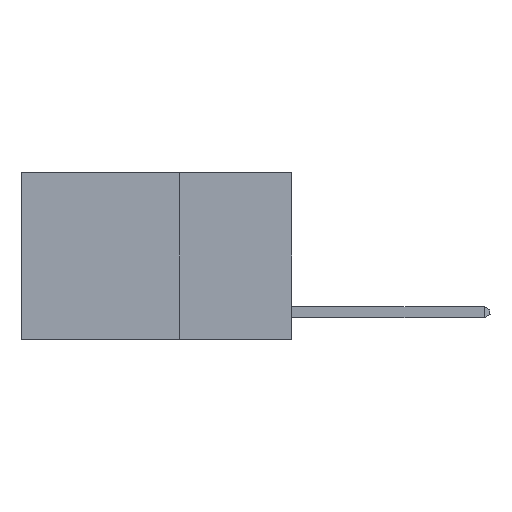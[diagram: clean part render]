
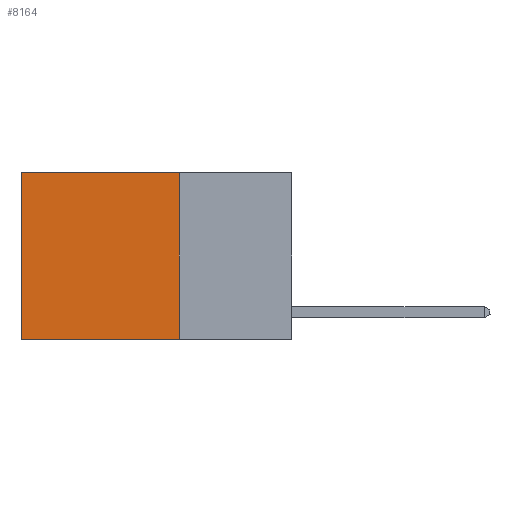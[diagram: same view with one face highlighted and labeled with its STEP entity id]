
A CAD part, left-side view. The second image highlights one B-rep face of the part: STEP entity #8164.
In plain terms, the highlighted planar face has unit normal (-1, 0, 0).
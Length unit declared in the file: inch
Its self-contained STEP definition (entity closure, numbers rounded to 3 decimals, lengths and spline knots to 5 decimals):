
#120 = VERTEX_POINT ( 'NONE', #10152 ) ;
#177 = VECTOR ( 'NONE', #1969, 39.37008 ) ;
#361 = VECTOR ( 'NONE', #2943, 39.37008 ) ;
#1296 = AXIS2_PLACEMENT_3D ( 'NONE', #7259, #12402, #7137 ) ;
#1969 = DIRECTION ( 'NONE',  ( 0., 0., -1. ) ) ;
#2112 = EDGE_CURVE ( 'NONE', #12924, #120, #5916, .T. ) ;
#2836 = DIRECTION ( 'NONE',  ( 0., 1., 0. ) ) ;
#2943 = DIRECTION ( 'NONE',  ( 0., 0., -1. ) ) ;
#3273 = EDGE_LOOP ( 'NONE', ( #9702, #4408, #4881, #5681 ) ) ;
#4176 = EDGE_CURVE ( 'NONE', #7712, #12924, #6089, .T. ) ;
#4379 = CARTESIAN_POINT ( 'NONE',  ( 0.2625, 0.25, 0. ) ) ;
#4408 = ORIENTED_EDGE ( 'NONE', *, *, #2112, .F. ) ;
#4881 = ORIENTED_EDGE ( 'NONE', *, *, #4176, .F. ) ;
#5681 = ORIENTED_EDGE ( 'NONE', *, *, #9122, .T. ) ;
#5916 = LINE ( 'NONE', #12054, #6511 ) ;
#6089 = LINE ( 'NONE', #12163, #361 ) ;
#6100 = CARTESIAN_POINT ( 'NONE',  ( 0.2625, 0.6, 0. ) ) ;
#6511 = VECTOR ( 'NONE', #2836, 39.37008 ) ;
#7137 = DIRECTION ( 'NONE',  ( 0., 0., -1. ) ) ;
#7259 = CARTESIAN_POINT ( 'NONE',  ( 0.2625, 0.25, 0. ) ) ;
#7391 = EDGE_CURVE ( 'NONE', #9214, #120, #10397, .T. ) ;
#7712 = VERTEX_POINT ( 'NONE', #11055 ) ;
#8164 = ADVANCED_FACE ( 'NONE', ( #9351 ), #13364, .F. ) ;
#8655 = LINE ( 'NONE', #4379, #12314 ) ;
#9122 = EDGE_CURVE ( 'NONE', #7712, #9214, #8655, .T. ) ;
#9214 = VERTEX_POINT ( 'NONE', #11081 ) ;
#9351 = FACE_OUTER_BOUND ( 'NONE', #3273, .T. ) ;
#9702 = ORIENTED_EDGE ( 'NONE', *, *, #7391, .T. ) ;
#10152 = CARTESIAN_POINT ( 'NONE',  ( 0.2625, 0.6, -0.37 ) ) ;
#10397 = LINE ( 'NONE', #6100, #177 ) ;
#10551 = DIRECTION ( 'NONE',  ( 0., 1., 0. ) ) ;
#10835 = CARTESIAN_POINT ( 'NONE',  ( 0.2625, 0.25, -0.37 ) ) ;
#11055 = CARTESIAN_POINT ( 'NONE',  ( 0.2625, 0.25, 0. ) ) ;
#11081 = CARTESIAN_POINT ( 'NONE',  ( 0.2625, 0.6, 0. ) ) ;
#12054 = CARTESIAN_POINT ( 'NONE',  ( 0.2625, 0.25, -0.37 ) ) ;
#12163 = CARTESIAN_POINT ( 'NONE',  ( 0.2625, 0.25, 0. ) ) ;
#12314 = VECTOR ( 'NONE', #10551, 39.37008 ) ;
#12402 = DIRECTION ( 'NONE',  ( 1., 0., 0. ) ) ;
#12924 = VERTEX_POINT ( 'NONE', #10835 ) ;
#13364 = PLANE ( 'NONE',  #1296 ) ;
